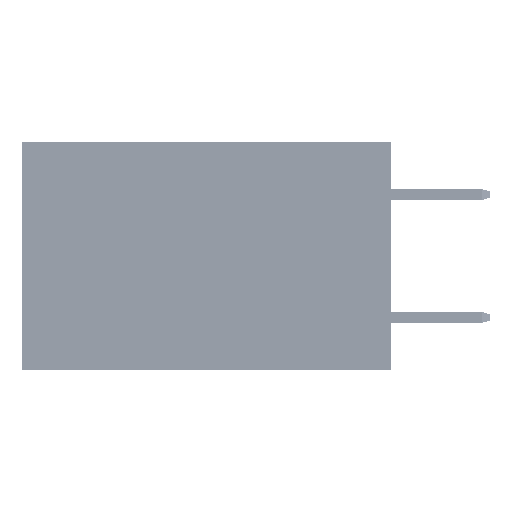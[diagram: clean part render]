
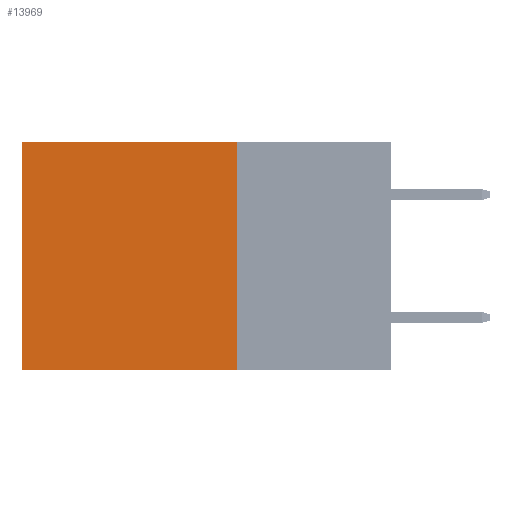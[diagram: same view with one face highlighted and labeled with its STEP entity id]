
A CAD part, left-side view. The second image highlights one B-rep face of the part: STEP entity #13969.
In plain terms, the highlighted planar face has unit normal (-1, 0, 0).
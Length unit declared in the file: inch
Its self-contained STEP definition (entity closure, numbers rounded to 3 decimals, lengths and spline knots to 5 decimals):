
#2527 = VERTEX_POINT ( 'NONE', #41208 ) ;
#3292 = LINE ( 'NONE', #7693, #4502 ) ;
#4502 = VECTOR ( 'NONE', #26558, 39.37008 ) ;
#6912 = EDGE_LOOP ( 'NONE', ( #30094, #22267, #31942, #8466 ) ) ;
#7693 = CARTESIAN_POINT ( 'NONE',  ( 0.2875, 0.25, 0. ) ) ;
#8466 = ORIENTED_EDGE ( 'NONE', *, *, #23244, .T. ) ;
#12827 = VERTEX_POINT ( 'NONE', #18568 ) ;
#13521 = FACE_OUTER_BOUND ( 'NONE', #6912, .T. ) ;
#13817 = VERTEX_POINT ( 'NONE', #20390 ) ;
#13969 = ADVANCED_FACE ( 'NONE', ( #13521 ), #25286, .F. ) ;
#14842 = DIRECTION ( 'NONE',  ( 0., 1., 0. ) ) ;
#14991 = EDGE_CURVE ( 'NONE', #13817, #2527, #3292, .T. ) ;
#15166 = CARTESIAN_POINT ( 'NONE',  ( 0.2875, 0.6, 0. ) ) ;
#15899 = LINE ( 'NONE', #15166, #33263 ) ;
#17758 = VECTOR ( 'NONE', #38163, 39.37008 ) ;
#18568 = CARTESIAN_POINT ( 'NONE',  ( 0.2875, 0.6, -0.37 ) ) ;
#20390 = CARTESIAN_POINT ( 'NONE',  ( 0.2875, 0.25, 0. ) ) ;
#20631 = DIRECTION ( 'NONE',  ( 0., 0., -1. ) ) ;
#22267 = ORIENTED_EDGE ( 'NONE', *, *, #39153, .F. ) ;
#23244 = EDGE_CURVE ( 'NONE', #13817, #41902, #26626, .T. ) ;
#24554 = CARTESIAN_POINT ( 'NONE',  ( 0.2875, 0.25, 0. ) ) ;
#24565 = VECTOR ( 'NONE', #14842, 39.37008 ) ;
#24623 = AXIS2_PLACEMENT_3D ( 'NONE', #24554, #39536, #20631 ) ;
#25286 = PLANE ( 'NONE',  #24623 ) ;
#26558 = DIRECTION ( 'NONE',  ( 0., 0., -1. ) ) ;
#26626 = LINE ( 'NONE', #30569, #17758 ) ;
#30094 = ORIENTED_EDGE ( 'NONE', *, *, #40033, .T. ) ;
#30569 = CARTESIAN_POINT ( 'NONE',  ( 0.2875, 0.25, 0. ) ) ;
#31942 = ORIENTED_EDGE ( 'NONE', *, *, #14991, .F. ) ;
#33263 = VECTOR ( 'NONE', #45097, 39.37008 ) ;
#38163 = DIRECTION ( 'NONE',  ( 0., 1., 0. ) ) ;
#39153 = EDGE_CURVE ( 'NONE', #2527, #12827, #44304, .T. ) ;
#39536 = DIRECTION ( 'NONE',  ( 1., 0., 0. ) ) ;
#40033 = EDGE_CURVE ( 'NONE', #41902, #12827, #15899, .T. ) ;
#41208 = CARTESIAN_POINT ( 'NONE',  ( 0.2875, 0.25, -0.37 ) ) ;
#41902 = VERTEX_POINT ( 'NONE', #45536 ) ;
#44304 = LINE ( 'NONE', #45030, #24565 ) ;
#45030 = CARTESIAN_POINT ( 'NONE',  ( 0.2875, 0.25, -0.37 ) ) ;
#45097 = DIRECTION ( 'NONE',  ( 0., 0., -1. ) ) ;
#45536 = CARTESIAN_POINT ( 'NONE',  ( 0.2875, 0.6, 0. ) ) ;
